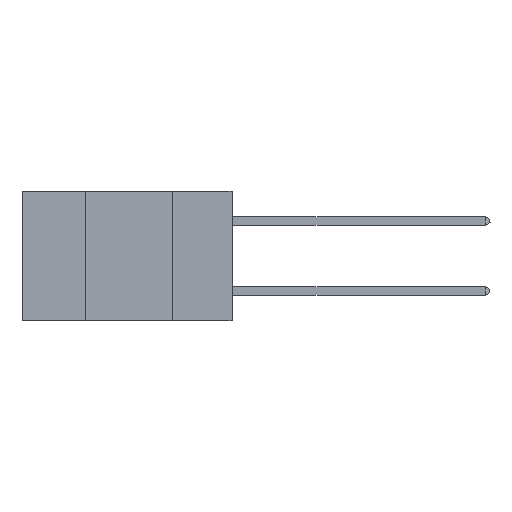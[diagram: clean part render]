
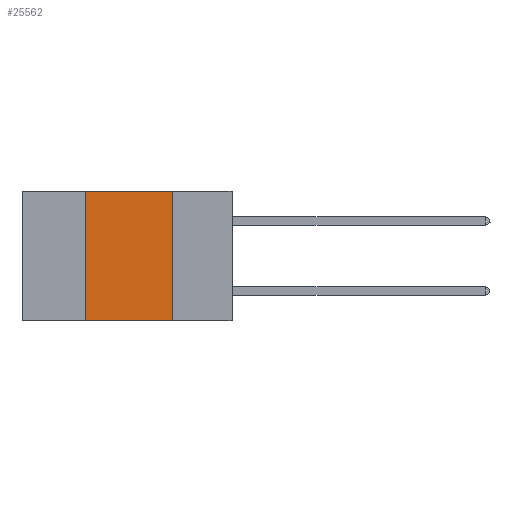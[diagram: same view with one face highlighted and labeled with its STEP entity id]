
A CAD part, left-side view. The second image highlights one B-rep face of the part: STEP entity #25562.
In plain terms, the highlighted planar face has unit normal (-1, 0, 0).
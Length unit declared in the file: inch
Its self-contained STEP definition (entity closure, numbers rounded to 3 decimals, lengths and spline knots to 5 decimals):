
#1095 = CARTESIAN_POINT ( 'NONE',  ( 0., 0.6, 0. ) ) ;
#1414 = CARTESIAN_POINT ( 'NONE',  ( 0., 0.17, 0. ) ) ;
#1524 = ORIENTED_EDGE ( 'NONE', *, *, #26024, .F. ) ;
#3055 = ORIENTED_EDGE ( 'NONE', *, *, #4497, .F. ) ;
#3134 = DIRECTION ( 'NONE',  ( 0., -1., 0. ) ) ;
#3865 = DIRECTION ( 'NONE',  ( 1., 0., 0. ) ) ;
#4497 = EDGE_CURVE ( 'NONE', #20616, #11199, #6042, .T. ) ;
#4665 = DIRECTION ( 'NONE',  ( 0., -1., 0. ) ) ;
#6042 = LINE ( 'NONE', #21090, #29310 ) ;
#6909 = VECTOR ( 'NONE', #4665, 39.37008 ) ;
#7354 = FACE_OUTER_BOUND ( 'NONE', #23630, .T. ) ;
#10222 = DIRECTION ( 'NONE',  ( 0., 0., 1. ) ) ;
#11199 = VERTEX_POINT ( 'NONE', #12593 ) ;
#12369 = PLANE ( 'NONE',  #20109 ) ;
#12593 = CARTESIAN_POINT ( 'NONE',  ( 0., 0.42, 0. ) ) ;
#13978 = CARTESIAN_POINT ( 'NONE',  ( 0., 0.17, -0.37 ) ) ;
#14573 = CARTESIAN_POINT ( 'NONE',  ( 0., 0.42, -0.37 ) ) ;
#14948 = LINE ( 'NONE', #30321, #23029 ) ;
#15496 = LINE ( 'NONE', #18259, #6909 ) ;
#17381 = VECTOR ( 'NONE', #18005, 39.37008 ) ;
#18005 = DIRECTION ( 'NONE',  ( 0., 0., -1. ) ) ;
#18259 = CARTESIAN_POINT ( 'NONE',  ( 0., 0.6, 0. ) ) ;
#19130 = EDGE_CURVE ( 'NONE', #20616, #20347, #14948, .T. ) ;
#20109 = AXIS2_PLACEMENT_3D ( 'NONE', #1095, #3865, #23603 ) ;
#20347 = VERTEX_POINT ( 'NONE', #13978 ) ;
#20616 = VERTEX_POINT ( 'NONE', #14573 ) ;
#21090 = CARTESIAN_POINT ( 'NONE',  ( 0., 0.42, 0. ) ) ;
#22895 = ORIENTED_EDGE ( 'NONE', *, *, #34407, .F. ) ;
#23029 = VECTOR ( 'NONE', #3134, 39.37008 ) ;
#23603 = DIRECTION ( 'NONE',  ( 0., 0., -1. ) ) ;
#23630 = EDGE_LOOP ( 'NONE', ( #22895, #1524, #3055, #25761 ) ) ;
#24694 = LINE ( 'NONE', #1414, #17381 ) ;
#25562 = ADVANCED_FACE ( 'NONE', ( #7354 ), #12369, .F. ) ;
#25761 = ORIENTED_EDGE ( 'NONE', *, *, #19130, .T. ) ;
#26024 = EDGE_CURVE ( 'NONE', #11199, #34856, #15496, .T. ) ;
#29310 = VECTOR ( 'NONE', #10222, 39.37008 ) ;
#30321 = CARTESIAN_POINT ( 'NONE',  ( 0., 0.6, -0.37 ) ) ;
#30599 = CARTESIAN_POINT ( 'NONE',  ( 0., 0.17, 0. ) ) ;
#34407 = EDGE_CURVE ( 'NONE', #34856, #20347, #24694, .T. ) ;
#34856 = VERTEX_POINT ( 'NONE', #30599 ) ;
